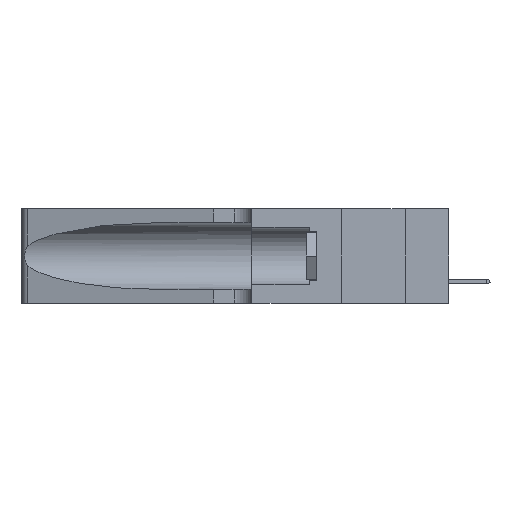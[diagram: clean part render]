
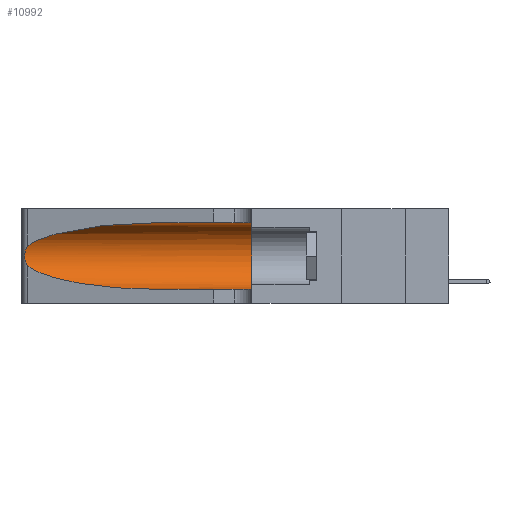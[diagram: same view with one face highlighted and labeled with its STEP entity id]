
A CAD part, left-side view. The second image highlights one B-rep face of the part: STEP entity #10992.
In plain terms, the highlighted cylindrical face has radius 3.308 mm (diameter 6.617 mm), a partial arc.
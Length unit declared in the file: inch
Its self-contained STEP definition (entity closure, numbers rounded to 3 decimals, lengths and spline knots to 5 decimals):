
#1146 = CARTESIAN_POINT ( 'NONE',  ( 0.25555, 1.22993, 0.14849 ) ) ;
#1186 = VERTEX_POINT ( 'NONE', #28164 ) ;
#1520 = ORIENTED_EDGE ( 'NONE', *, *, #6328, .T. ) ;
#3402 = CARTESIAN_POINT ( 'NONE',  ( 0.25789, 1.23486, 0.15765 ) ) ;
#3773 = CARTESIAN_POINT ( 'NONE',  ( 0.25487, 1.22718, 0.14631 ) ) ;
#3912 = VERTEX_POINT ( 'NONE', #26217 ) ;
#4228 = DIRECTION ( 'NONE',  ( 0., -1., 0. ) ) ;
#4536 = VERTEX_POINT ( 'NONE', #29605 ) ;
#5956 = CARTESIAN_POINT ( 'NONE',  ( 0.25555, 1.22994, 0.2215 ) ) ;
#6065 = ORIENTED_EDGE ( 'NONE', *, *, #28975, .T. ) ;
#6328 = EDGE_CURVE ( 'NONE', #16923, #11116, #9055, .T. ) ;
#6341 = EDGE_CURVE ( 'NONE', #3912, #11264, #19780, .T. ) ;
#6575 = CYLINDRICAL_SURFACE ( 'NONE', #23587, 0.13025 ) ;
#6626 =( BOUNDED_CURVE ( )  B_SPLINE_CURVE ( 3, ( #22850, #15790, #13229, #8790 ),
 .UNSPECIFIED., .F., .F. ) 
 B_SPLINE_CURVE_WITH_KNOTS ( ( 4, 4 ),
 ( 1.5708, 2.84003 ),
 .UNSPECIFIED. ) 
 CURVE ( )  GEOMETRIC_REPRESENTATION_ITEM ( )  RATIONAL_B_SPLINE_CURVE ( ( 1., 0.87, 0.87, 1. ) ) 
 REPRESENTATION_ITEM ( '' )  );
#7550 = CARTESIAN_POINT ( 'NONE',  ( 0.25487, 1.22718, 0.14631 ) ) ;
#8010 = CARTESIAN_POINT ( 'NONE',  ( 0.25639, 1.23184, 0.21858 ) ) ;
#8109 = CARTESIAN_POINT ( 'NONE',  ( 0.25854, 1.2359, 0.20912 ) ) ;
#8271 = CARTESIAN_POINT ( 'NONE',  ( 0.18966, 0.96281, 0.05475 ) ) ;
#8278 = VECTOR ( 'NONE', #27814, 39.37008 ) ;
#8762 = CIRCLE ( 'NONE', #10681, 0.13025 ) ;
#8790 = CARTESIAN_POINT ( 'NONE',  ( 0.25487, 1.22718, 0.22369 ) ) ;
#9055 = B_SPLINE_CURVE_WITH_KNOTS ( 'NONE', 3,
 ( #17662, #5956, #8010, #24795, #8109, #22367, #29167, #27136, #10359, #10472, #3402, #19781, #1146, #17561 ),
 .UNSPECIFIED., .F., .F.,
 ( 4, 2, 2, 2, 2, 2, 4 ),
 ( 0., 0.00027, 0.00053, 0.00107, 0.0016, 0.00187, 0.00214 ),
 .UNSPECIFIED. ) ;
#9152 = VECTOR ( 'NONE', #4228, 39.37008 ) ;
#9780 =( BOUNDED_CURVE ( )  B_SPLINE_CURVE ( 3, ( #3773, #20146, #8271, #22535 ),
 .UNSPECIFIED., .F., .F. ) 
 B_SPLINE_CURVE_WITH_KNOTS ( ( 4, 4 ),
 ( 3.44316, 4.71239 ),
 .UNSPECIFIED. ) 
 CURVE ( )  GEOMETRIC_REPRESENTATION_ITEM ( )  RATIONAL_B_SPLINE_CURVE ( ( 1., 0.87, 0.87, 1. ) ) 
 REPRESENTATION_ITEM ( '' )  );
#10359 = CARTESIAN_POINT ( 'NONE',  ( 0.26017, 1.23833, 0.17102 ) ) ;
#10472 = CARTESIAN_POINT ( 'NONE',  ( 0.25856, 1.23593, 0.16098 ) ) ;
#10667 = EDGE_LOOP ( 'NONE', ( #6065, #1520, #20315, #14247, #28338, #29403 ) ) ;
#10681 = AXIS2_PLACEMENT_3D ( 'NONE', #22951, #29655, #15591 ) ;
#10992 = ADVANCED_FACE ( 'NONE', ( #19365 ), #6575, .F. ) ;
#11116 = VERTEX_POINT ( 'NONE', #7550 ) ;
#11227 = CARTESIAN_POINT ( 'NONE',  ( 0.1305, 1.61858, 0.185 ) ) ;
#11264 = VERTEX_POINT ( 'NONE', #28032 ) ;
#11677 = CARTESIAN_POINT ( 'NONE',  ( 0.1305, 1.61858, 0.05475 ) ) ;
#13229 = CARTESIAN_POINT ( 'NONE',  ( 0.2373, 1.15595, 0.28018 ) ) ;
#14247 = ORIENTED_EDGE ( 'NONE', *, *, #21645, .T. ) ;
#14700 = DIRECTION ( 'NONE',  ( 0., 0., -1. ) ) ;
#14835 = DIRECTION ( 'NONE',  ( 0., -1., 0. ) ) ;
#15198 = CARTESIAN_POINT ( 'NONE',  ( 0.1305, 1.61858, 0.31525 ) ) ;
#15591 = DIRECTION ( 'NONE',  ( 0., 0., 1. ) ) ;
#15790 = CARTESIAN_POINT ( 'NONE',  ( 0.18966, 0.96281, 0.31525 ) ) ;
#16923 = VERTEX_POINT ( 'NONE', #17541 ) ;
#17541 = CARTESIAN_POINT ( 'NONE',  ( 0.25487, 1.22718, 0.22369 ) ) ;
#17561 = CARTESIAN_POINT ( 'NONE',  ( 0.25487, 1.22718, 0.14631 ) ) ;
#17662 = CARTESIAN_POINT ( 'NONE',  ( 0.25487, 1.22718, 0.22369 ) ) ;
#19365 = FACE_OUTER_BOUND ( 'NONE', #10667, .T. ) ;
#19780 = LINE ( 'NONE', #15198, #9152 ) ;
#19781 = CARTESIAN_POINT ( 'NONE',  ( 0.25639, 1.23186, 0.15144 ) ) ;
#20146 = CARTESIAN_POINT ( 'NONE',  ( 0.2373, 1.15595, 0.08982 ) ) ;
#20315 = ORIENTED_EDGE ( 'NONE', *, *, #23585, .T. ) ;
#21645 = EDGE_CURVE ( 'NONE', #1186, #4536, #28015, .T. ) ;
#22367 = CARTESIAN_POINT ( 'NONE',  ( 0.26018, 1.23835, 0.19895 ) ) ;
#22535 = CARTESIAN_POINT ( 'NONE',  ( 0.1305, 0.72297, 0.05475 ) ) ;
#22850 = CARTESIAN_POINT ( 'NONE',  ( 0.1305, 0.72297, 0.31525 ) ) ;
#22951 = CARTESIAN_POINT ( 'NONE',  ( 0.1305, 0.35, 0.185 ) ) ;
#23585 = EDGE_CURVE ( 'NONE', #11116, #1186, #9780, .T. ) ;
#23587 = AXIS2_PLACEMENT_3D ( 'NONE', #11227, #14835, #14700 ) ;
#24795 = CARTESIAN_POINT ( 'NONE',  ( 0.25787, 1.23484, 0.2124 ) ) ;
#26217 = CARTESIAN_POINT ( 'NONE',  ( 0.1305, 0.72297, 0.31525 ) ) ;
#27136 = CARTESIAN_POINT ( 'NONE',  ( 0.26075, 1.23896, 0.178 ) ) ;
#27814 = DIRECTION ( 'NONE',  ( 0., -1., 0. ) ) ;
#28015 = LINE ( 'NONE', #11677, #8278 ) ;
#28032 = CARTESIAN_POINT ( 'NONE',  ( 0.1305, 0.35, 0.31525 ) ) ;
#28164 = CARTESIAN_POINT ( 'NONE',  ( 0.1305, 0.72297, 0.05475 ) ) ;
#28338 = ORIENTED_EDGE ( 'NONE', *, *, #28957, .F. ) ;
#28957 = EDGE_CURVE ( 'NONE', #11264, #4536, #8762, .T. ) ;
#28975 = EDGE_CURVE ( 'NONE', #3912, #16923, #6626, .T. ) ;
#29167 = CARTESIAN_POINT ( 'NONE',  ( 0.26075, 1.23896, 0.19203 ) ) ;
#29403 = ORIENTED_EDGE ( 'NONE', *, *, #6341, .F. ) ;
#29605 = CARTESIAN_POINT ( 'NONE',  ( 0.1305, 0.35, 0.05475 ) ) ;
#29655 = DIRECTION ( 'NONE',  ( 0., 1., 0. ) ) ;
